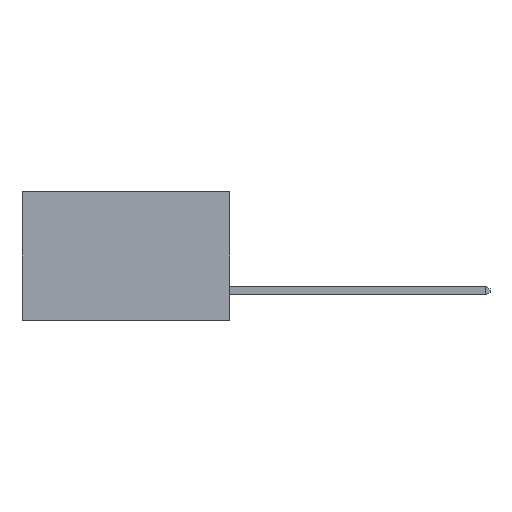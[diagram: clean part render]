
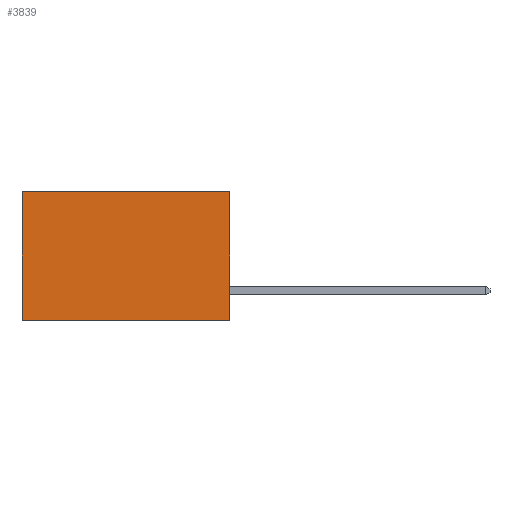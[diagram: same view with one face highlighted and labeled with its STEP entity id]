
A CAD part, left-side view. The second image highlights one B-rep face of the part: STEP entity #3839.
In plain terms, the highlighted planar face has unit normal (-1, 0, 0).
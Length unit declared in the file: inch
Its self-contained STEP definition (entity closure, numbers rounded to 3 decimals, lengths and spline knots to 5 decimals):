
#14 = DIRECTION ( 'NONE',  ( 1., 0., 0. ) ) ;
#93 = DIRECTION ( 'NONE',  ( 0., 0., -1. ) ) ;
#522 = EDGE_CURVE ( 'NONE', #10023, #9661, #4280, .T. ) ;
#763 = EDGE_CURVE ( 'NONE', #10023, #12585, #10141, .T. ) ;
#966 = VECTOR ( 'NONE', #2553, 39.37008 ) ;
#1866 = DIRECTION ( 'NONE',  ( 0., 0., -1. ) ) ;
#2024 = CARTESIAN_POINT ( 'NONE',  ( 0.298, 0., 0. ) ) ;
#2269 = DIRECTION ( 'NONE',  ( 0., 1., 0. ) ) ;
#2553 = DIRECTION ( 'NONE',  ( 0., 0., -1. ) ) ;
#2622 = EDGE_CURVE ( 'NONE', #12585, #6670, #8651, .T. ) ;
#2656 = CARTESIAN_POINT ( 'NONE',  ( 0.298, 0.6, -0.37 ) ) ;
#2726 = CARTESIAN_POINT ( 'NONE',  ( 0.298, 0., 0. ) ) ;
#2796 = VECTOR ( 'NONE', #2269, 39.37008 ) ;
#3349 = CARTESIAN_POINT ( 'NONE',  ( 0.298, 0., 0. ) ) ;
#3381 = PLANE ( 'NONE',  #7309 ) ;
#3839 = ADVANCED_FACE ( 'NONE', ( #11129 ), #3381, .F. ) ;
#3933 = VECTOR ( 'NONE', #6741, 39.37008 ) ;
#4183 = EDGE_LOOP ( 'NONE', ( #9302, #6979, #11170, #7561 ) ) ;
#4280 = LINE ( 'NONE', #6149, #3933 ) ;
#4374 = EDGE_CURVE ( 'NONE', #9661, #6670, #6511, .T. ) ;
#5159 = CARTESIAN_POINT ( 'NONE',  ( 0.298, 0., -0.37 ) ) ;
#6149 = CARTESIAN_POINT ( 'NONE',  ( 0.298, 0., 0. ) ) ;
#6358 = CARTESIAN_POINT ( 'NONE',  ( 0.298, 0., -0.37 ) ) ;
#6511 = LINE ( 'NONE', #11253, #966 ) ;
#6670 = VERTEX_POINT ( 'NONE', #2656 ) ;
#6741 = DIRECTION ( 'NONE',  ( 0., 1., 0. ) ) ;
#6979 = ORIENTED_EDGE ( 'NONE', *, *, #2622, .F. ) ;
#7309 = AXIS2_PLACEMENT_3D ( 'NONE', #3349, #14, #93 ) ;
#7561 = ORIENTED_EDGE ( 'NONE', *, *, #522, .T. ) ;
#8651 = LINE ( 'NONE', #5159, #2796 ) ;
#9302 = ORIENTED_EDGE ( 'NONE', *, *, #4374, .T. ) ;
#9661 = VERTEX_POINT ( 'NONE', #11302 ) ;
#10023 = VERTEX_POINT ( 'NONE', #2726 ) ;
#10141 = LINE ( 'NONE', #2024, #12360 ) ;
#11129 = FACE_OUTER_BOUND ( 'NONE', #4183, .T. ) ;
#11170 = ORIENTED_EDGE ( 'NONE', *, *, #763, .F. ) ;
#11253 = CARTESIAN_POINT ( 'NONE',  ( 0.298, 0.6, 0. ) ) ;
#11302 = CARTESIAN_POINT ( 'NONE',  ( 0.298, 0.6, 0. ) ) ;
#12360 = VECTOR ( 'NONE', #1866, 39.37008 ) ;
#12585 = VERTEX_POINT ( 'NONE', #6358 ) ;
